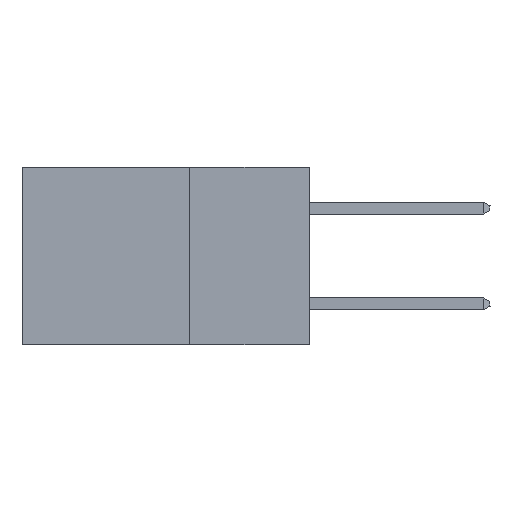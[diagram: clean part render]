
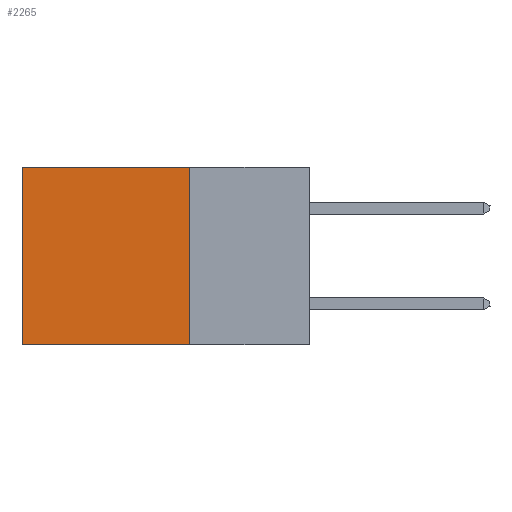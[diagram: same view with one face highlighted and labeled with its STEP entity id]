
A CAD part, left-side view. The second image highlights one B-rep face of the part: STEP entity #2265.
In plain terms, the highlighted planar face has unit normal (-1, 0, 0).
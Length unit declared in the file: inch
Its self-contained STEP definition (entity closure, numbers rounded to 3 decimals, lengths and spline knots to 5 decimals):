
#1033 = EDGE_CURVE ( 'NONE', #24103, #10130, #20515, .T. ) ;
#2194 = DIRECTION ( 'NONE',  ( 0., 1., 0. ) ) ;
#2265 = ADVANCED_FACE ( 'NONE', ( #10608 ), #10892, .F. ) ;
#2476 = CARTESIAN_POINT ( 'NONE',  ( 0.2875, 0.25, 0. ) ) ;
#5249 = EDGE_CURVE ( 'NONE', #13786, #13167, #25716, .T. ) ;
#5382 = ORIENTED_EDGE ( 'NONE', *, *, #31699, .F. ) ;
#5934 = VECTOR ( 'NONE', #30112, 39.37008 ) ;
#7001 = ORIENTED_EDGE ( 'NONE', *, *, #1033, .T. ) ;
#7765 = DIRECTION ( 'NONE',  ( 0., 0., -1. ) ) ;
#10130 = VERTEX_POINT ( 'NONE', #30676 ) ;
#10608 = FACE_OUTER_BOUND ( 'NONE', #20524, .T. ) ;
#10892 = PLANE ( 'NONE',  #31899 ) ;
#10978 = CARTESIAN_POINT ( 'NONE',  ( 0.2875, 0.25, 0. ) ) ;
#11839 = CARTESIAN_POINT ( 'NONE',  ( 0.2875, 0.25, -0.37 ) ) ;
#13167 = VERTEX_POINT ( 'NONE', #21313 ) ;
#13181 = CARTESIAN_POINT ( 'NONE',  ( 0.2875, 0.25, -0.37 ) ) ;
#13786 = VERTEX_POINT ( 'NONE', #11839 ) ;
#14455 = DIRECTION ( 'NONE',  ( 0., 0., -1. ) ) ;
#17159 = VECTOR ( 'NONE', #2194, 39.37008 ) ;
#19898 = CARTESIAN_POINT ( 'NONE',  ( 0.2875, 0.25, 0. ) ) ;
#20515 = LINE ( 'NONE', #10978, #5934 ) ;
#20524 = EDGE_LOOP ( 'NONE', ( #25731, #31943, #5382, #7001 ) ) ;
#21313 = CARTESIAN_POINT ( 'NONE',  ( 0.2875, 0.6, -0.37 ) ) ;
#21669 = CARTESIAN_POINT ( 'NONE',  ( 0.2875, 0.6, 0. ) ) ;
#21679 = DIRECTION ( 'NONE',  ( 0., 0., -1. ) ) ;
#23037 = LINE ( 'NONE', #21669, #25620 ) ;
#24103 = VERTEX_POINT ( 'NONE', #30172 ) ;
#24402 = DIRECTION ( 'NONE',  ( 1., 0., 0. ) ) ;
#24706 = EDGE_CURVE ( 'NONE', #10130, #13167, #23037, .T. ) ;
#25620 = VECTOR ( 'NONE', #7765, 39.37008 ) ;
#25716 = LINE ( 'NONE', #13181, #17159 ) ;
#25731 = ORIENTED_EDGE ( 'NONE', *, *, #24706, .T. ) ;
#30112 = DIRECTION ( 'NONE',  ( 0., 1., 0. ) ) ;
#30172 = CARTESIAN_POINT ( 'NONE',  ( 0.2875, 0.25, 0. ) ) ;
#30590 = VECTOR ( 'NONE', #14455, 39.37008 ) ;
#30676 = CARTESIAN_POINT ( 'NONE',  ( 0.2875, 0.6, 0. ) ) ;
#31699 = EDGE_CURVE ( 'NONE', #24103, #13786, #32740, .T. ) ;
#31899 = AXIS2_PLACEMENT_3D ( 'NONE', #2476, #24402, #21679 ) ;
#31943 = ORIENTED_EDGE ( 'NONE', *, *, #5249, .F. ) ;
#32740 = LINE ( 'NONE', #19898, #30590 ) ;
